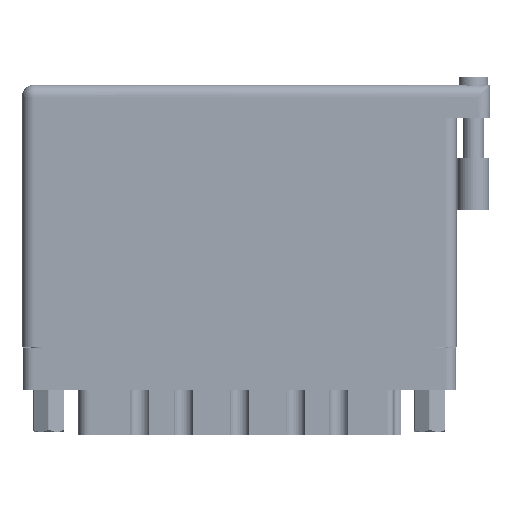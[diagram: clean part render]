
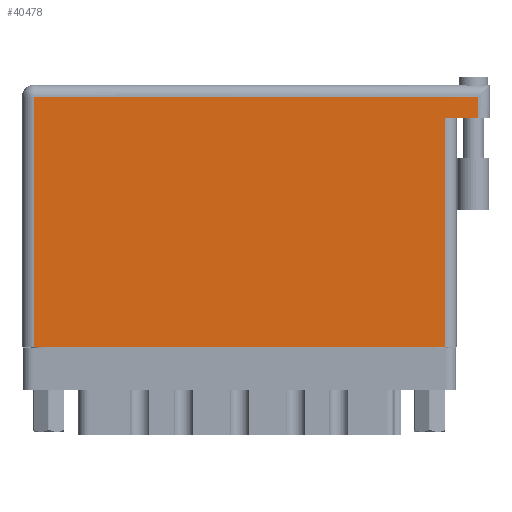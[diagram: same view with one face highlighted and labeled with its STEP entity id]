
A CAD part, front view. The second image highlights one B-rep face of the part: STEP entity #40478.
In plain terms, the highlighted face is planar.
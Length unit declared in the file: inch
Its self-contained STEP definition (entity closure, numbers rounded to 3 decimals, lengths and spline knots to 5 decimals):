
#207 = AXIS2_PLACEMENT_3D ( 'NONE', #27973, #46943, #8884 ) ;
#2454 = ORIENTED_EDGE ( 'NONE', *, *, #7295, .T. ) ;
#2496 = ORIENTED_EDGE ( 'NONE', *, *, #38067, .T. ) ;
#2907 = LINE ( 'NONE', #17930, #25338 ) ;
#3157 = EDGE_CURVE ( 'NONE', #36788, #36662, #2907, .T. ) ;
#5438 = EDGE_CURVE ( 'NONE', #36736, #55474, #40731, .T. ) ;
#7295 = EDGE_CURVE ( 'NONE', #55474, #36662, #31725, .T. ) ;
#7903 = CARTESIAN_POINT ( 'NONE',  ( 2.73, 1.566, 0. ) ) ;
#8023 = CARTESIAN_POINT ( 'NONE',  ( 2.73, 1.369, 0. ) ) ;
#8884 = DIRECTION ( 'NONE',  ( -1., 0., 0. ) ) ;
#9059 = ORIENTED_EDGE ( 'NONE', *, *, #25304, .T. ) ;
#11756 = VERTEX_POINT ( 'NONE', #25957 ) ;
#13822 = ORIENTED_EDGE ( 'NONE', *, *, #3157, .F. ) ;
#13967 = FACE_OUTER_BOUND ( 'NONE', #38495, .T. ) ;
#15295 = VECTOR ( 'NONE', #41360, 39.37008 ) ;
#15672 = CARTESIAN_POINT ( 'NONE',  ( 2.53, 0., 0. ) ) ;
#16284 = LINE ( 'NONE', #7903, #43915 ) ;
#17930 = CARTESIAN_POINT ( 'NONE',  ( 2.8, 1.369, 0. ) ) ;
#18941 = CARTESIAN_POINT ( 'NONE',  ( 2.53, 1.369, 0. ) ) ;
#21647 = ORIENTED_EDGE ( 'NONE', *, *, #5438, .T. ) ;
#21939 = CARTESIAN_POINT ( 'NONE',  ( 0., 0., 0. ) ) ;
#21990 = VECTOR ( 'NONE', #32271, 39.37008 ) ;
#23827 = ORIENTED_EDGE ( 'NONE', *, *, #32217, .T. ) ;
#23886 = VECTOR ( 'NONE', #49120, 39.37008 ) ;
#25304 = EDGE_CURVE ( 'NONE', #11756, #51670, #26772, .T. ) ;
#25338 = VECTOR ( 'NONE', #47731, 39.37008 ) ;
#25957 = CARTESIAN_POINT ( 'NONE',  ( 2.73, 1.496, 0. ) ) ;
#26648 = DIRECTION ( 'NONE',  ( -1., 0., 0. ) ) ;
#26772 = LINE ( 'NONE', #45426, #61232 ) ;
#27973 = CARTESIAN_POINT ( 'NONE',  ( 0., 1.566, 0. ) ) ;
#31725 = LINE ( 'NONE', #56130, #21990 ) ;
#32157 = DIRECTION ( 'NONE',  ( 0., 1., 0. ) ) ;
#32217 = EDGE_CURVE ( 'NONE', #36788, #11756, #16284, .T. ) ;
#32271 = DIRECTION ( 'NONE',  ( 0., 1., 0. ) ) ;
#36662 = VERTEX_POINT ( 'NONE', #18941 ) ;
#36736 = VERTEX_POINT ( 'NONE', #48226 ) ;
#36788 = VERTEX_POINT ( 'NONE', #8023 ) ;
#38067 = EDGE_CURVE ( 'NONE', #51670, #36736, #53097, .T. ) ;
#38495 = EDGE_LOOP ( 'NONE', ( #21647, #2454, #13822, #23827, #9059, #2496 ) ) ;
#40478 = ADVANCED_FACE ( 'NONE', ( #13967 ), #51805, .F. ) ;
#40731 = LINE ( 'NONE', #21939, #15295 ) ;
#41360 = DIRECTION ( 'NONE',  ( 1., 0., 0. ) ) ;
#43915 = VECTOR ( 'NONE', #32157, 39.37008 ) ;
#45426 = CARTESIAN_POINT ( 'NONE',  ( 0., 1.496, 0. ) ) ;
#46943 = DIRECTION ( 'NONE',  ( 0., 0., -1. ) ) ;
#47731 = DIRECTION ( 'NONE',  ( -1., 0., 0. ) ) ;
#48226 = CARTESIAN_POINT ( 'NONE',  ( 0.07, 0., 0. ) ) ;
#49120 = DIRECTION ( 'NONE',  ( 0., -1., 0. ) ) ;
#51670 = VERTEX_POINT ( 'NONE', #56018 ) ;
#51805 = PLANE ( 'NONE',  #207 ) ;
#53097 = LINE ( 'NONE', #58551, #23886 ) ;
#55474 = VERTEX_POINT ( 'NONE', #15672 ) ;
#56018 = CARTESIAN_POINT ( 'NONE',  ( 0.07, 1.496, 0. ) ) ;
#56130 = CARTESIAN_POINT ( 'NONE',  ( 2.53, 1.369, 0. ) ) ;
#58551 = CARTESIAN_POINT ( 'NONE',  ( 0.07, 0., 0. ) ) ;
#61232 = VECTOR ( 'NONE', #26648, 39.37008 ) ;
